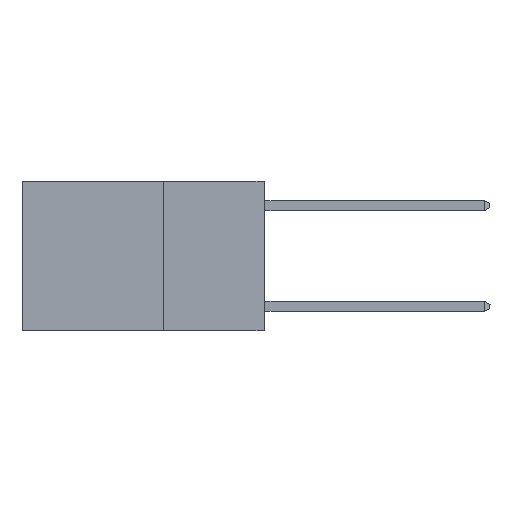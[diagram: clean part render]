
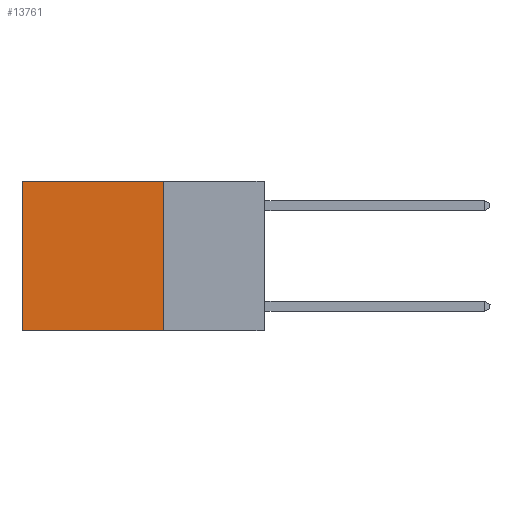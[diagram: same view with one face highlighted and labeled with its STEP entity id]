
A CAD part, left-side view. The second image highlights one B-rep face of the part: STEP entity #13761.
In plain terms, the highlighted planar face has unit normal (-1, 0, 0).
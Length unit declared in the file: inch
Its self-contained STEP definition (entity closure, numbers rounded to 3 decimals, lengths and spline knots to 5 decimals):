
#181 = DIRECTION ( 'NONE',  ( 0., 0., -1. ) ) ;
#985 = EDGE_CURVE ( 'NONE', #20522, #12364, #14563, .T. ) ;
#1170 = DIRECTION ( 'NONE',  ( 0., 1., 0. ) ) ;
#1825 = DIRECTION ( 'NONE',  ( 1., 0., 0. ) ) ;
#1892 = EDGE_CURVE ( 'NONE', #12364, #14786, #2037, .T. ) ;
#2037 = LINE ( 'NONE', #7043, #14746 ) ;
#2143 = LINE ( 'NONE', #7287, #10790 ) ;
#2223 = EDGE_CURVE ( 'NONE', #22259, #14786, #10141, .T. ) ;
#2387 = ORIENTED_EDGE ( 'NONE', *, *, #2223, .F. ) ;
#2963 = CARTESIAN_POINT ( 'NONE',  ( 0.2625, 0.25, -0.37 ) ) ;
#3097 = ORIENTED_EDGE ( 'NONE', *, *, #5806, .F. ) ;
#4542 = VECTOR ( 'NONE', #1170, 39.37008 ) ;
#5806 = EDGE_CURVE ( 'NONE', #20522, #22259, #2143, .T. ) ;
#6058 = CARTESIAN_POINT ( 'NONE',  ( 0.2625, 0.6, -0.37 ) ) ;
#6941 = CARTESIAN_POINT ( 'NONE',  ( 0.2625, 0.25, 0. ) ) ;
#7043 = CARTESIAN_POINT ( 'NONE',  ( 0.2625, 0.6, 0. ) ) ;
#7287 = CARTESIAN_POINT ( 'NONE',  ( 0.2625, 0.25, 0. ) ) ;
#8210 = CARTESIAN_POINT ( 'NONE',  ( 0.2625, 0.25, -0.37 ) ) ;
#8643 = DIRECTION ( 'NONE',  ( 0., 1., 0. ) ) ;
#8761 = DIRECTION ( 'NONE',  ( 0., 0., -1. ) ) ;
#9977 = VECTOR ( 'NONE', #8643, 39.37008 ) ;
#10141 = LINE ( 'NONE', #2963, #4542 ) ;
#10790 = VECTOR ( 'NONE', #181, 39.37008 ) ;
#12201 = PLANE ( 'NONE',  #19960 ) ;
#12364 = VERTEX_POINT ( 'NONE', #20614 ) ;
#13761 = ADVANCED_FACE ( 'NONE', ( #17836 ), #12201, .F. ) ;
#13931 = DIRECTION ( 'NONE',  ( 0., 0., -1. ) ) ;
#14391 = EDGE_LOOP ( 'NONE', ( #16413, #2387, #3097, #20502 ) ) ;
#14563 = LINE ( 'NONE', #6941, #9977 ) ;
#14746 = VECTOR ( 'NONE', #8761, 39.37008 ) ;
#14786 = VERTEX_POINT ( 'NONE', #6058 ) ;
#16413 = ORIENTED_EDGE ( 'NONE', *, *, #1892, .T. ) ;
#17078 = CARTESIAN_POINT ( 'NONE',  ( 0.2625, 0.25, 0. ) ) ;
#17836 = FACE_OUTER_BOUND ( 'NONE', #14391, .T. ) ;
#18971 = CARTESIAN_POINT ( 'NONE',  ( 0.2625, 0.25, 0. ) ) ;
#19960 = AXIS2_PLACEMENT_3D ( 'NONE', #18971, #1825, #13931 ) ;
#20502 = ORIENTED_EDGE ( 'NONE', *, *, #985, .T. ) ;
#20522 = VERTEX_POINT ( 'NONE', #17078 ) ;
#20614 = CARTESIAN_POINT ( 'NONE',  ( 0.2625, 0.6, 0. ) ) ;
#22259 = VERTEX_POINT ( 'NONE', #8210 ) ;
